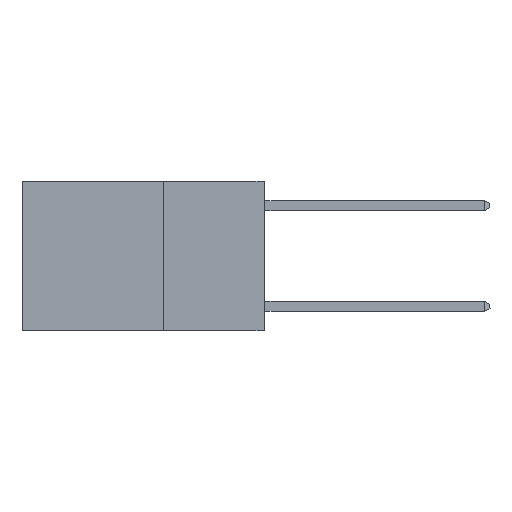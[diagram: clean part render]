
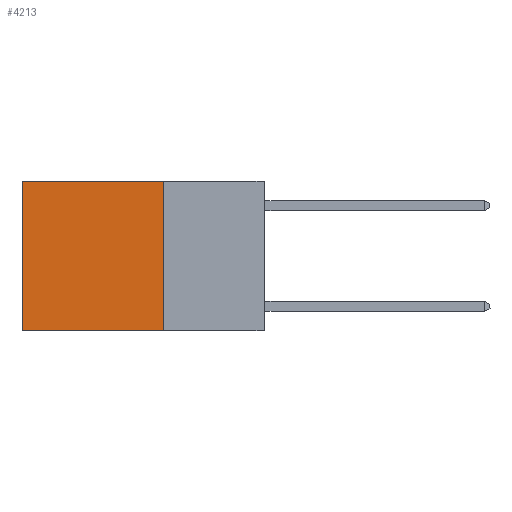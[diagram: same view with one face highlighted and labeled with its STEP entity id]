
A CAD part, left-side view. The second image highlights one B-rep face of the part: STEP entity #4213.
In plain terms, the highlighted planar face has unit normal (-1, 0, 0).
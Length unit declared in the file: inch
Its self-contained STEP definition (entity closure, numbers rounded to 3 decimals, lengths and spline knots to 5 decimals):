
#448 = DIRECTION ( 'NONE',  ( 0., 0., -1. ) ) ;
#718 = VECTOR ( 'NONE', #3188, 39.37008 ) ;
#856 = PLANE ( 'NONE',  #5354 ) ;
#891 = CARTESIAN_POINT ( 'NONE',  ( 0.2625, 0.25, -0.37 ) ) ;
#1121 = EDGE_CURVE ( 'NONE', #7560, #7604, #7216, .T. ) ;
#1276 = ORIENTED_EDGE ( 'NONE', *, *, #11187, .T. ) ;
#1430 = EDGE_LOOP ( 'NONE', ( #1276, #7051, #8451, #3871 ) ) ;
#2328 = CARTESIAN_POINT ( 'NONE',  ( 0.2625, 0.25, 0. ) ) ;
#3188 = DIRECTION ( 'NONE',  ( 0., 1., 0. ) ) ;
#3264 = LINE ( 'NONE', #7870, #718 ) ;
#3651 = EDGE_CURVE ( 'NONE', #7604, #10587, #5044, .T. ) ;
#3871 = ORIENTED_EDGE ( 'NONE', *, *, #7253, .T. ) ;
#4213 = ADVANCED_FACE ( 'NONE', ( #6410 ), #856, .F. ) ;
#4352 = VECTOR ( 'NONE', #448, 39.37008 ) ;
#4531 = CARTESIAN_POINT ( 'NONE',  ( 0.2625, 0.25, 0. ) ) ;
#5044 = LINE ( 'NONE', #9034, #9556 ) ;
#5197 = DIRECTION ( 'NONE',  ( 0., 0., -1. ) ) ;
#5354 = AXIS2_PLACEMENT_3D ( 'NONE', #6615, #6712, #8173 ) ;
#6410 = FACE_OUTER_BOUND ( 'NONE', #1430, .T. ) ;
#6606 = CARTESIAN_POINT ( 'NONE',  ( 0.2625, 0.6, 0. ) ) ;
#6615 = CARTESIAN_POINT ( 'NONE',  ( 0.2625, 0.25, 0. ) ) ;
#6712 = DIRECTION ( 'NONE',  ( 1., 0., 0. ) ) ;
#6966 = LINE ( 'NONE', #11230, #8992 ) ;
#7051 = ORIENTED_EDGE ( 'NONE', *, *, #3651, .F. ) ;
#7216 = LINE ( 'NONE', #2328, #4352 ) ;
#7253 = EDGE_CURVE ( 'NONE', #7560, #10429, #3264, .T. ) ;
#7560 = VERTEX_POINT ( 'NONE', #4531 ) ;
#7604 = VERTEX_POINT ( 'NONE', #891 ) ;
#7645 = CARTESIAN_POINT ( 'NONE',  ( 0.2625, 0.6, -0.37 ) ) ;
#7870 = CARTESIAN_POINT ( 'NONE',  ( 0.2625, 0.25, 0. ) ) ;
#8173 = DIRECTION ( 'NONE',  ( 0., 0., -1. ) ) ;
#8451 = ORIENTED_EDGE ( 'NONE', *, *, #1121, .F. ) ;
#8992 = VECTOR ( 'NONE', #5197, 39.37008 ) ;
#9034 = CARTESIAN_POINT ( 'NONE',  ( 0.2625, 0.25, -0.37 ) ) ;
#9556 = VECTOR ( 'NONE', #11468, 39.37008 ) ;
#10429 = VERTEX_POINT ( 'NONE', #6606 ) ;
#10587 = VERTEX_POINT ( 'NONE', #7645 ) ;
#11187 = EDGE_CURVE ( 'NONE', #10429, #10587, #6966, .T. ) ;
#11230 = CARTESIAN_POINT ( 'NONE',  ( 0.2625, 0.6, 0. ) ) ;
#11468 = DIRECTION ( 'NONE',  ( 0., 1., 0. ) ) ;
